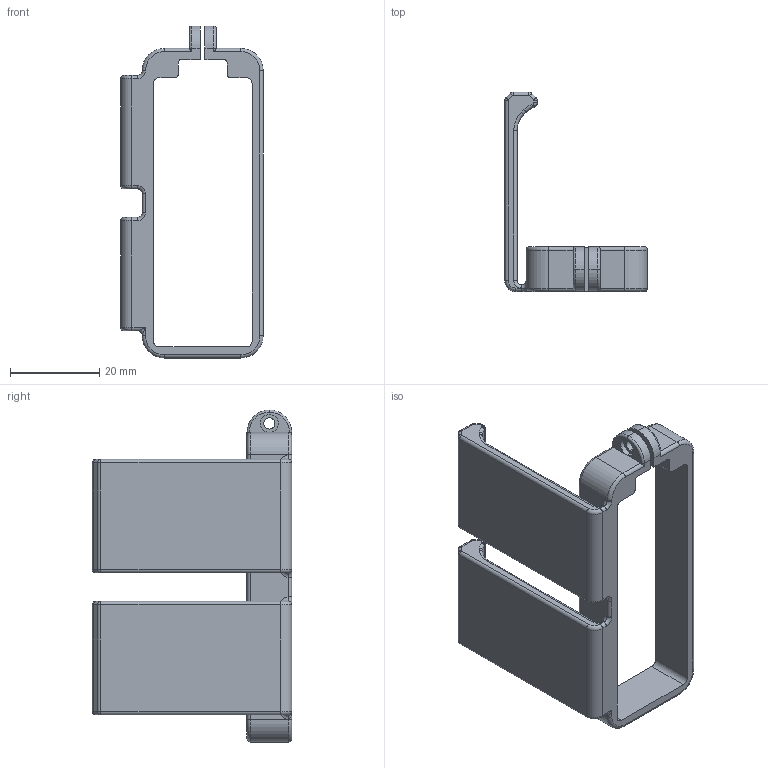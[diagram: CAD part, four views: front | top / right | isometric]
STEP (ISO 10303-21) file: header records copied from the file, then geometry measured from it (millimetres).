
FILE_DESCRIPTION (( 'STEP AP214' ), '1' );
FILE_NAME ('Bolted_Clamp.STEP', '2013-12-11T18:02:40', ( 'elpi' ), ( '' ), 'SwSTEP 2.0', 'SolidWorks 2013', '' );
FILE_SCHEMA (( 'AUTOMOTIVE_DESIGN' ));
Length unit declared in the file: millimetre
Products named in the file (1): Bolted_Clamp
Bounding box: 31.86 x 44.6 x 74.26 mm (x, y, z)
Volume: 12157.5 mm3; surface area: 10068.4 mm2
Topology: 1 solids, 1 shells, 192 faces, 464 edges, 273 vertices
Faces by surface type: cylinder 94, torus 55, plane 42, bspline 1
Entity records: 5682 total; most frequent: DIRECTION 1091, CARTESIAN_POINT 1007, ORIENTED_EDGE 926, EDGE_CURVE 463, AXIS2_PLACEMENT_3D 443, VERTEX_POINT 273, CIRCLE 251, VECTOR 205
